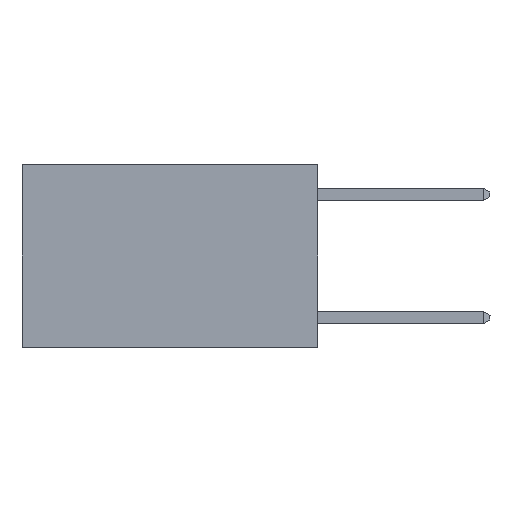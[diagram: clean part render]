
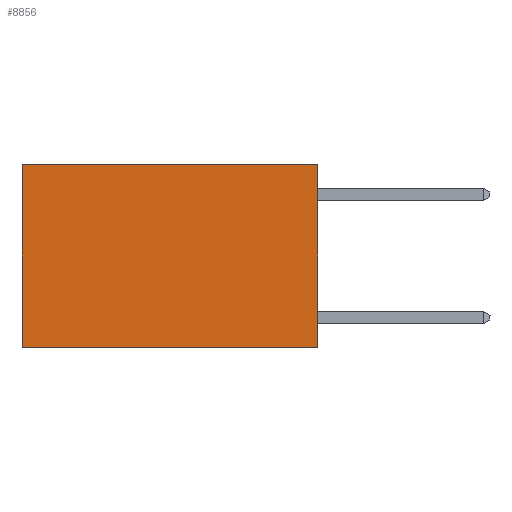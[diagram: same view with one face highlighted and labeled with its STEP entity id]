
A CAD part, left-side view. The second image highlights one B-rep face of the part: STEP entity #8856.
In plain terms, the highlighted planar face has unit normal (-1, 0, 0).
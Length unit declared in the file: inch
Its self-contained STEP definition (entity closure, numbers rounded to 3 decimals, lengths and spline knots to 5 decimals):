
#55 = CARTESIAN_POINT ( 'NONE',  ( 0.2625, 0., 0. ) ) ;
#233 = CARTESIAN_POINT ( 'NONE',  ( 0.2625, 0., -0.37 ) ) ;
#355 = VECTOR ( 'NONE', #17858, 39.37008 ) ;
#755 = CARTESIAN_POINT ( 'NONE',  ( 0.2625, 0.6, 0. ) ) ;
#972 = VERTEX_POINT ( 'NONE', #55 ) ;
#1714 = DIRECTION ( 'NONE',  ( 1., 0., 0. ) ) ;
#2261 = DIRECTION ( 'NONE',  ( 0., 0., -1. ) ) ;
#5468 = DIRECTION ( 'NONE',  ( 0., 1., 0. ) ) ;
#6099 = PLANE ( 'NONE',  #12250 ) ;
#6849 = EDGE_CURVE ( 'NONE', #972, #10693, #8194, .T. ) ;
#7092 = EDGE_CURVE ( 'NONE', #16643, #17137, #12981, .T. ) ;
#7177 = EDGE_CURVE ( 'NONE', #972, #16643, #7256, .T. ) ;
#7256 = LINE ( 'NONE', #10375, #14512 ) ;
#7883 = FACE_OUTER_BOUND ( 'NONE', #9051, .T. ) ;
#8194 = LINE ( 'NONE', #10617, #355 ) ;
#8856 = ADVANCED_FACE ( 'NONE', ( #7883 ), #6099, .F. ) ;
#9051 = EDGE_LOOP ( 'NONE', ( #13803, #12287, #14986, #14887 ) ) ;
#9095 = VECTOR ( 'NONE', #5468, 39.37008 ) ;
#10375 = CARTESIAN_POINT ( 'NONE',  ( 0.2625, 0., 0. ) ) ;
#10617 = CARTESIAN_POINT ( 'NONE',  ( 0.2625, 0., 0. ) ) ;
#10693 = VERTEX_POINT ( 'NONE', #14312 ) ;
#11850 = DIRECTION ( 'NONE',  ( 0., 0., -1. ) ) ;
#11981 = DIRECTION ( 'NONE',  ( 0., 0., -1. ) ) ;
#12250 = AXIS2_PLACEMENT_3D ( 'NONE', #17675, #1714, #11981 ) ;
#12287 = ORIENTED_EDGE ( 'NONE', *, *, #7092, .F. ) ;
#12812 = CARTESIAN_POINT ( 'NONE',  ( 0.2625, 0., -0.37 ) ) ;
#12981 = LINE ( 'NONE', #12812, #9095 ) ;
#13591 = CARTESIAN_POINT ( 'NONE',  ( 0.2625, 0.6, -0.37 ) ) ;
#13803 = ORIENTED_EDGE ( 'NONE', *, *, #16276, .T. ) ;
#14312 = CARTESIAN_POINT ( 'NONE',  ( 0.2625, 0.6, 0. ) ) ;
#14512 = VECTOR ( 'NONE', #11850, 39.37008 ) ;
#14887 = ORIENTED_EDGE ( 'NONE', *, *, #6849, .T. ) ;
#14986 = ORIENTED_EDGE ( 'NONE', *, *, #7177, .F. ) ;
#16276 = EDGE_CURVE ( 'NONE', #10693, #17137, #17338, .T. ) ;
#16643 = VERTEX_POINT ( 'NONE', #233 ) ;
#17137 = VERTEX_POINT ( 'NONE', #13591 ) ;
#17338 = LINE ( 'NONE', #755, #17766 ) ;
#17675 = CARTESIAN_POINT ( 'NONE',  ( 0.2625, 0., 0. ) ) ;
#17766 = VECTOR ( 'NONE', #2261, 39.37008 ) ;
#17858 = DIRECTION ( 'NONE',  ( 0., 1., 0. ) ) ;
